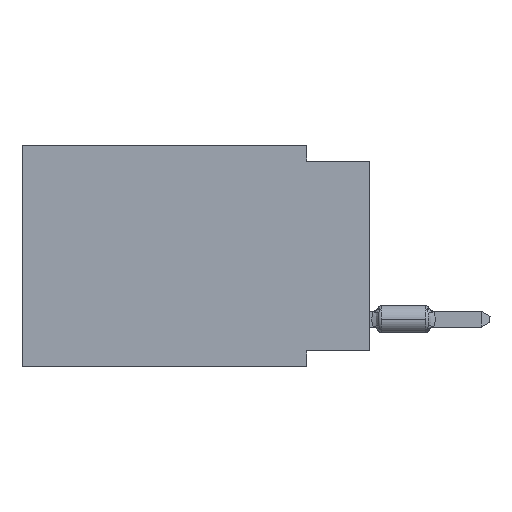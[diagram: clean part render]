
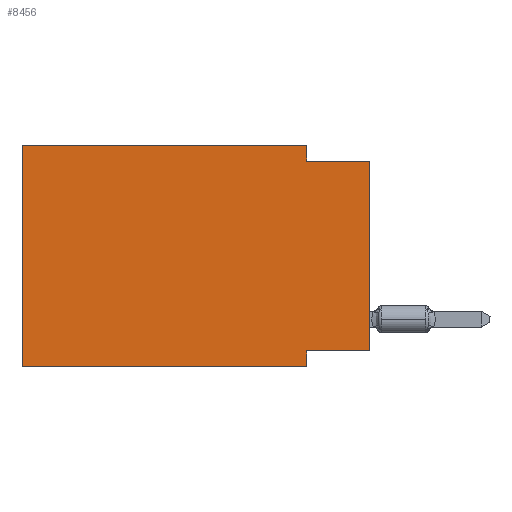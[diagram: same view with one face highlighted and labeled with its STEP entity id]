
A CAD part, left-side view. The second image highlights one B-rep face of the part: STEP entity #8456.
In plain terms, the highlighted planar face has unit normal (-1, 0, 0).
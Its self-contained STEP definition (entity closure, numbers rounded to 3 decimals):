
#722 = CARTESIAN_POINT ( 'NONE',  ( 0., 13.97, 0. ) ) ;
#1049 = CARTESIAN_POINT ( 'NONE',  ( 0., 2.54, -8.89 ) ) ;
#1133 = DIRECTION ( 'NONE',  ( 0., 0., 1. ) ) ;
#1203 = EDGE_CURVE ( 'NONE', #9536, #3339, #21486, .T. ) ;
#1520 = LINE ( 'NONE', #1049, #2607 ) ;
#2607 = VECTOR ( 'NONE', #15702, 1000. ) ;
#2996 = DIRECTION ( 'NONE',  ( 0., 0., -1. ) ) ;
#3050 = EDGE_CURVE ( 'NONE', #3339, #24844, #1520, .T. ) ;
#3339 = VERTEX_POINT ( 'NONE', #26331 ) ;
#4295 = CARTESIAN_POINT ( 'NONE',  ( 0., 13.97, 0. ) ) ;
#4422 = ORIENTED_EDGE ( 'NONE', *, *, #16651, .F. ) ;
#5405 = ORIENTED_EDGE ( 'NONE', *, *, #3050, .F. ) ;
#5413 = ORIENTED_EDGE ( 'NONE', *, *, #1203, .F. ) ;
#5803 = EDGE_LOOP ( 'NONE', ( #17342, #26364, #10888, #4422, #22828, #24724, #5405, #5413 ) ) ;
#6576 = VECTOR ( 'NONE', #26850, 1000. ) ;
#6997 = PLANE ( 'NONE',  #15783 ) ;
#7601 = EDGE_CURVE ( 'NONE', #12033, #9215, #9684, .T. ) ;
#8102 = VECTOR ( 'NONE', #2996, 1000. ) ;
#8294 = LINE ( 'NONE', #23096, #10493 ) ;
#8456 = ADVANCED_FACE ( 'NONE', ( #26107 ), #6997, .F. ) ;
#9215 = VERTEX_POINT ( 'NONE', #16639 ) ;
#9536 = VERTEX_POINT ( 'NONE', #15368 ) ;
#9684 = LINE ( 'NONE', #29560, #6576 ) ;
#10117 = CARTESIAN_POINT ( 'NONE',  ( 0., 13.97, -8.89 ) ) ;
#10269 = CARTESIAN_POINT ( 'NONE',  ( 0., 13.97, -8.89 ) ) ;
#10493 = VECTOR ( 'NONE', #1133, 1000. ) ;
#10888 = ORIENTED_EDGE ( 'NONE', *, *, #18966, .F. ) ;
#12033 = VERTEX_POINT ( 'NONE', #12559 ) ;
#12559 = CARTESIAN_POINT ( 'NONE',  ( 0., 2.54, -0.635 ) ) ;
#12888 = CARTESIAN_POINT ( 'NONE',  ( 0., 2.54, 0. ) ) ;
#13480 = CARTESIAN_POINT ( 'NONE',  ( 0., 0., 0. ) ) ;
#14010 = DIRECTION ( 'NONE',  ( 1., 0., 0. ) ) ;
#14158 = CARTESIAN_POINT ( 'NONE',  ( 0., 0., -8.255 ) ) ;
#15032 = LINE ( 'NONE', #10269, #20297 ) ;
#15054 = DIRECTION ( 'NONE',  ( 0., -1., 0. ) ) ;
#15368 = CARTESIAN_POINT ( 'NONE',  ( 0., 0., -8.255 ) ) ;
#15702 = DIRECTION ( 'NONE',  ( 0., 0., -1. ) ) ;
#15783 = AXIS2_PLACEMENT_3D ( 'NONE', #4295, #14010, #26424 ) ;
#16512 = VERTEX_POINT ( 'NONE', #10117 ) ;
#16639 = CARTESIAN_POINT ( 'NONE',  ( 0., 0., -0.635 ) ) ;
#16651 = EDGE_CURVE ( 'NONE', #30601, #28130, #20312, .T. ) ;
#17268 = VECTOR ( 'NONE', #22703, 1000. ) ;
#17342 = ORIENTED_EDGE ( 'NONE', *, *, #28543, .T. ) ;
#18966 = EDGE_CURVE ( 'NONE', #28130, #12033, #29414, .T. ) ;
#20297 = VECTOR ( 'NONE', #24903, 1000. ) ;
#20312 = LINE ( 'NONE', #722, #28305 ) ;
#20577 = CARTESIAN_POINT ( 'NONE',  ( 0., 13.97, 0. ) ) ;
#21045 = CARTESIAN_POINT ( 'NONE',  ( 0., 2.54, -8.89 ) ) ;
#21425 = EDGE_CURVE ( 'NONE', #16512, #30601, #8294, .T. ) ;
#21486 = LINE ( 'NONE', #14158, #25929 ) ;
#22423 = CARTESIAN_POINT ( 'NONE',  ( 0., 2.54, 0. ) ) ;
#22703 = DIRECTION ( 'NONE',  ( 0., 0., 1. ) ) ;
#22828 = ORIENTED_EDGE ( 'NONE', *, *, #21425, .F. ) ;
#22868 = LINE ( 'NONE', #13480, #17268 ) ;
#23096 = CARTESIAN_POINT ( 'NONE',  ( 0., 13.97, 0. ) ) ;
#23692 = DIRECTION ( 'NONE',  ( 0., 1., 0. ) ) ;
#24724 = ORIENTED_EDGE ( 'NONE', *, *, #27744, .T. ) ;
#24844 = VERTEX_POINT ( 'NONE', #21045 ) ;
#24903 = DIRECTION ( 'NONE',  ( 0., -1., 0. ) ) ;
#25929 = VECTOR ( 'NONE', #23692, 1000. ) ;
#26107 = FACE_OUTER_BOUND ( 'NONE', #5803, .T. ) ;
#26331 = CARTESIAN_POINT ( 'NONE',  ( 0., 2.54, -8.255 ) ) ;
#26364 = ORIENTED_EDGE ( 'NONE', *, *, #7601, .F. ) ;
#26424 = DIRECTION ( 'NONE',  ( 0., 0., -1. ) ) ;
#26850 = DIRECTION ( 'NONE',  ( 0., -1., 0. ) ) ;
#27744 = EDGE_CURVE ( 'NONE', #16512, #24844, #15032, .T. ) ;
#28130 = VERTEX_POINT ( 'NONE', #12888 ) ;
#28305 = VECTOR ( 'NONE', #15054, 1000. ) ;
#28543 = EDGE_CURVE ( 'NONE', #9536, #9215, #22868, .T. ) ;
#29414 = LINE ( 'NONE', #22423, #8102 ) ;
#29560 = CARTESIAN_POINT ( 'NONE',  ( 0., 0., -0.635 ) ) ;
#30601 = VERTEX_POINT ( 'NONE', #20577 ) ;
